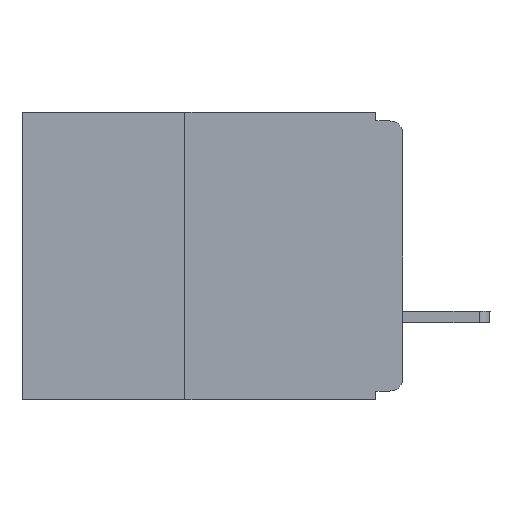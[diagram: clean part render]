
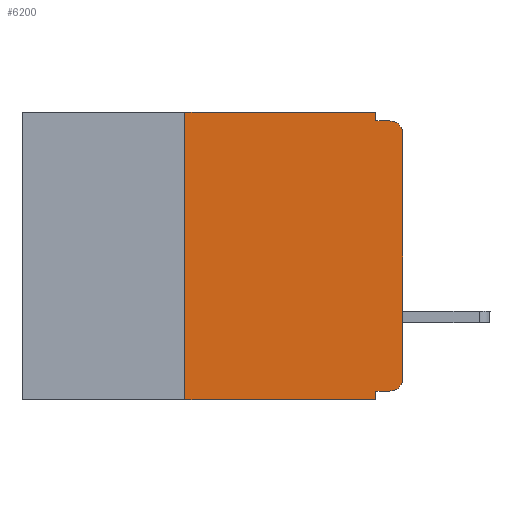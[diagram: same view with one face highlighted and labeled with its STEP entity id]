
A CAD part, left-side view. The second image highlights one B-rep face of the part: STEP entity #6200.
In plain terms, the highlighted planar face has unit normal (-1, 0, 0).
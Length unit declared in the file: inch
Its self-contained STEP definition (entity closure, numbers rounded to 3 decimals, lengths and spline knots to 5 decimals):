
#68 = VERTEX_POINT ( 'NONE', #14938 ) ;
#103 = ORIENTED_EDGE ( 'NONE', *, *, #5722, .T. ) ;
#143 = DIRECTION ( 'NONE',  ( 0., 0., 1. ) ) ;
#434 = LINE ( 'NONE', #714, #8640 ) ;
#613 = DIRECTION ( 'NONE',  ( 0., -1., 0. ) ) ;
#714 = CARTESIAN_POINT ( 'NONE',  ( 0., 0.437, -0.33 ) ) ;
#731 = ORIENTED_EDGE ( 'NONE', *, *, #2151, .F. ) ;
#739 = DIRECTION ( 'NONE',  ( 0., 0., -1. ) ) ;
#800 = EDGE_CURVE ( 'NONE', #12855, #13352, #12087, .T. ) ;
#909 = VERTEX_POINT ( 'NONE', #3155 ) ;
#1190 = CIRCLE ( 'NONE', #11502, 0.015 ) ;
#1379 = CARTESIAN_POINT ( 'NONE',  ( 0., 0., -0.025 ) ) ;
#1388 = ORIENTED_EDGE ( 'NONE', *, *, #12883, .T. ) ;
#1502 = LINE ( 'NONE', #11110, #11722 ) ;
#1923 = CARTESIAN_POINT ( 'NONE',  ( 0., 0.015, -0.01 ) ) ;
#2128 = ORIENTED_EDGE ( 'NONE', *, *, #7323, .F. ) ;
#2151 = EDGE_CURVE ( 'NONE', #10200, #7252, #5969, .T. ) ;
#2154 = EDGE_CURVE ( 'NONE', #6023, #12560, #9112, .T. ) ;
#2161 = DIRECTION ( 'NONE',  ( -1., 0., 0. ) ) ;
#2180 = CARTESIAN_POINT ( 'NONE',  ( 0., 0.015, -0.32 ) ) ;
#2326 = VERTEX_POINT ( 'NONE', #13421 ) ;
#2375 = VECTOR ( 'NONE', #3527, 39.37008 ) ;
#2383 = DIRECTION ( 'NONE',  ( 0., 0., -1. ) ) ;
#2604 = LINE ( 'NONE', #11876, #2970 ) ;
#2766 = DIRECTION ( 'NONE',  ( -1., 0., 0. ) ) ;
#2970 = VECTOR ( 'NONE', #143, 39.37008 ) ;
#3155 = CARTESIAN_POINT ( 'NONE',  ( 0., 0.25, 0. ) ) ;
#3527 = DIRECTION ( 'NONE',  ( 0., 1., 0. ) ) ;
#3586 = CARTESIAN_POINT ( 'NONE',  ( 0., 0.031, -0.32 ) ) ;
#3646 = VERTEX_POINT ( 'NONE', #13954 ) ;
#4071 = EDGE_CURVE ( 'NONE', #12560, #13352, #5580, .T. ) ;
#4628 = CARTESIAN_POINT ( 'NONE',  ( 0., 0.031, 0. ) ) ;
#4913 = EDGE_CURVE ( 'NONE', #3646, #12855, #14883, .T. ) ;
#5288 = LINE ( 'NONE', #10169, #14240 ) ;
#5580 = LINE ( 'NONE', #12674, #10540 ) ;
#5722 = EDGE_CURVE ( 'NONE', #10200, #3646, #1190, .T. ) ;
#5949 = DIRECTION ( 'NONE',  ( 0., 0., 1. ) ) ;
#5969 = LINE ( 'NONE', #12532, #2375 ) ;
#6023 = VERTEX_POINT ( 'NONE', #7973 ) ;
#6200 = ADVANCED_FACE ( 'NONE', ( #9935 ), #8216, .F. ) ;
#6713 = EDGE_LOOP ( 'NONE', ( #14261, #13802, #9325, #7588, #10385, #2128, #1388, #14487, #731, #103 ) ) ;
#7252 = VERTEX_POINT ( 'NONE', #3586 ) ;
#7323 = EDGE_CURVE ( 'NONE', #68, #909, #2604, .T. ) ;
#7520 = EDGE_CURVE ( 'NONE', #909, #6023, #1502, .T. ) ;
#7588 = ORIENTED_EDGE ( 'NONE', *, *, #2154, .F. ) ;
#7973 = CARTESIAN_POINT ( 'NONE',  ( 0., 0.031, 0. ) ) ;
#8216 = PLANE ( 'NONE',  #8368 ) ;
#8368 = AXIS2_PLACEMENT_3D ( 'NONE', #10606, #9536, #11679 ) ;
#8640 = VECTOR ( 'NONE', #13515, 39.37008 ) ;
#9112 = LINE ( 'NONE', #4628, #10930 ) ;
#9305 = DIRECTION ( 'NONE',  ( 0., -1., 0. ) ) ;
#9325 = ORIENTED_EDGE ( 'NONE', *, *, #4071, .F. ) ;
#9536 = DIRECTION ( 'NONE',  ( 1., 0., 0. ) ) ;
#9817 = CARTESIAN_POINT ( 'NONE',  ( 0., 0.015, -0.025 ) ) ;
#9935 = FACE_OUTER_BOUND ( 'NONE', #6713, .T. ) ;
#10169 = CARTESIAN_POINT ( 'NONE',  ( 0., 0.031, -0.33 ) ) ;
#10200 = VERTEX_POINT ( 'NONE', #2180 ) ;
#10385 = ORIENTED_EDGE ( 'NONE', *, *, #7520, .F. ) ;
#10540 = VECTOR ( 'NONE', #9305, 39.37008 ) ;
#10606 = CARTESIAN_POINT ( 'NONE',  ( 0., 0.437, 0. ) ) ;
#10930 = VECTOR ( 'NONE', #2383, 39.37008 ) ;
#10933 = DIRECTION ( 'NONE',  ( 0., 0., -1. ) ) ;
#11110 = CARTESIAN_POINT ( 'NONE',  ( 0., 0.437, 0. ) ) ;
#11332 = DIRECTION ( 'NONE',  ( 0., 0., -1. ) ) ;
#11502 = AXIS2_PLACEMENT_3D ( 'NONE', #12621, #2161, #11332 ) ;
#11679 = DIRECTION ( 'NONE',  ( 0., 0., -1. ) ) ;
#11722 = VECTOR ( 'NONE', #613, 39.37008 ) ;
#11876 = CARTESIAN_POINT ( 'NONE',  ( 0., 0.25, -0.33 ) ) ;
#11954 = CARTESIAN_POINT ( 'NONE',  ( 0., 0., 0. ) ) ;
#12087 = CIRCLE ( 'NONE', #12832, 0.015 ) ;
#12532 = CARTESIAN_POINT ( 'NONE',  ( 0., 0., -0.32 ) ) ;
#12560 = VERTEX_POINT ( 'NONE', #13730 ) ;
#12621 = CARTESIAN_POINT ( 'NONE',  ( 0., 0.015, -0.305 ) ) ;
#12674 = CARTESIAN_POINT ( 'NONE',  ( 0., 0., -0.01 ) ) ;
#12832 = AXIS2_PLACEMENT_3D ( 'NONE', #9817, #2766, #10933 ) ;
#12855 = VERTEX_POINT ( 'NONE', #1379 ) ;
#12883 = EDGE_CURVE ( 'NONE', #68, #2326, #434, .T. ) ;
#13352 = VERTEX_POINT ( 'NONE', #1923 ) ;
#13421 = CARTESIAN_POINT ( 'NONE',  ( 0., 0.031, -0.33 ) ) ;
#13515 = DIRECTION ( 'NONE',  ( 0., -1., 0. ) ) ;
#13730 = CARTESIAN_POINT ( 'NONE',  ( 0., 0.031, -0.01 ) ) ;
#13802 = ORIENTED_EDGE ( 'NONE', *, *, #800, .T. ) ;
#13954 = CARTESIAN_POINT ( 'NONE',  ( 0., 0., -0.305 ) ) ;
#13971 = VECTOR ( 'NONE', #5949, 39.37008 ) ;
#14240 = VECTOR ( 'NONE', #739, 39.37008 ) ;
#14261 = ORIENTED_EDGE ( 'NONE', *, *, #4913, .T. ) ;
#14311 = EDGE_CURVE ( 'NONE', #7252, #2326, #5288, .T. ) ;
#14487 = ORIENTED_EDGE ( 'NONE', *, *, #14311, .F. ) ;
#14883 = LINE ( 'NONE', #11954, #13971 ) ;
#14938 = CARTESIAN_POINT ( 'NONE',  ( 0., 0.25, -0.33 ) ) ;
